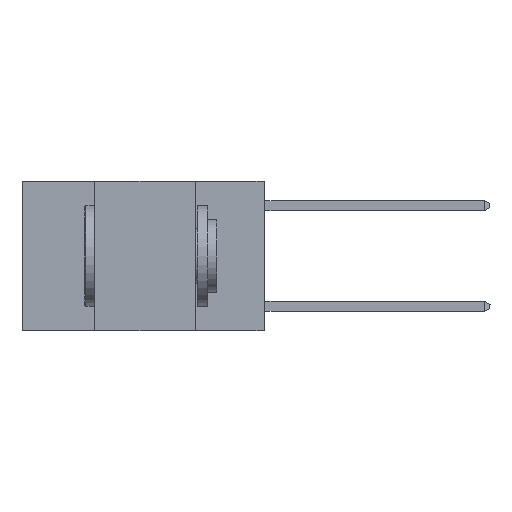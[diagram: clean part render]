
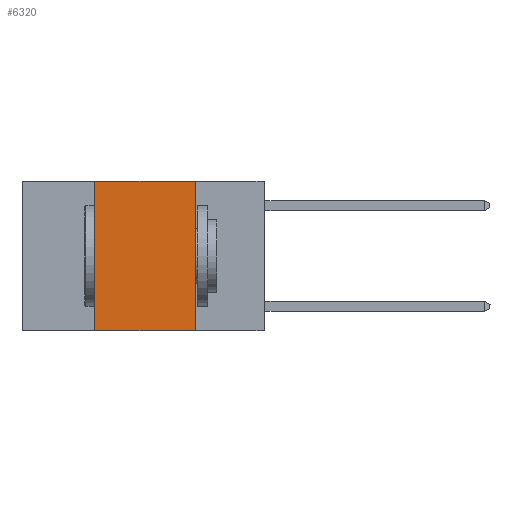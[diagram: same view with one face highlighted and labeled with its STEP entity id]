
A CAD part, left-side view. The second image highlights one B-rep face of the part: STEP entity #6320.
In plain terms, the highlighted planar face has unit normal (-1, 0, 0).
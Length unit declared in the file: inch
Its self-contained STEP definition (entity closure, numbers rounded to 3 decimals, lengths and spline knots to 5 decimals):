
#85 = VERTEX_POINT ( 'NONE', #10490 ) ;
#444 = DIRECTION ( 'NONE',  ( 0., 0., 1. ) ) ;
#3487 = EDGE_CURVE ( 'NONE', #22617, #15120, #13695, .T. ) ;
#5264 = CARTESIAN_POINT ( 'NONE',  ( 0., 0.42, 0. ) ) ;
#6052 = DIRECTION ( 'NONE',  ( 0., 0., -1. ) ) ;
#6320 = ADVANCED_FACE ( 'NONE', ( #25575 ), #9406, .F. ) ;
#7021 = CARTESIAN_POINT ( 'NONE',  ( 0., 0.6, 0. ) ) ;
#7198 = VECTOR ( 'NONE', #7482, 39.37008 ) ;
#7482 = DIRECTION ( 'NONE',  ( 0., -1., 0. ) ) ;
#8416 = CARTESIAN_POINT ( 'NONE',  ( 0., 0.6, 0. ) ) ;
#8564 = VECTOR ( 'NONE', #22892, 39.37008 ) ;
#9406 = PLANE ( 'NONE',  #19676 ) ;
#9510 = DIRECTION ( 'NONE',  ( 0., 0., -1. ) ) ;
#9922 = VECTOR ( 'NONE', #6052, 39.37008 ) ;
#10490 = CARTESIAN_POINT ( 'NONE',  ( 0., 0.17, 0. ) ) ;
#12734 = LINE ( 'NONE', #8416, #8564 ) ;
#13312 = CARTESIAN_POINT ( 'NONE',  ( 0., 0.17, 0. ) ) ;
#13695 = LINE ( 'NONE', #24418, #7198 ) ;
#15120 = VERTEX_POINT ( 'NONE', #24151 ) ;
#16175 = EDGE_CURVE ( 'NONE', #22973, #85, #12734, .T. ) ;
#16579 = EDGE_CURVE ( 'NONE', #22617, #22973, #19876, .T. ) ;
#17135 = ORIENTED_EDGE ( 'NONE', *, *, #16175, .F. ) ;
#17879 = ORIENTED_EDGE ( 'NONE', *, *, #16579, .F. ) ;
#19676 = AXIS2_PLACEMENT_3D ( 'NONE', #7021, #23963, #9510 ) ;
#19876 = LINE ( 'NONE', #5264, #25532 ) ;
#22008 = LINE ( 'NONE', #13312, #9922 ) ;
#22018 = ORIENTED_EDGE ( 'NONE', *, *, #29453, .F. ) ;
#22617 = VERTEX_POINT ( 'NONE', #30393 ) ;
#22892 = DIRECTION ( 'NONE',  ( 0., -1., 0. ) ) ;
#22973 = VERTEX_POINT ( 'NONE', #26907 ) ;
#23963 = DIRECTION ( 'NONE',  ( 1., 0., 0. ) ) ;
#24151 = CARTESIAN_POINT ( 'NONE',  ( 0., 0.17, -0.37 ) ) ;
#24350 = EDGE_LOOP ( 'NONE', ( #22018, #17135, #17879, #25033 ) ) ;
#24418 = CARTESIAN_POINT ( 'NONE',  ( 0., 0.6, -0.37 ) ) ;
#25033 = ORIENTED_EDGE ( 'NONE', *, *, #3487, .T. ) ;
#25532 = VECTOR ( 'NONE', #444, 39.37008 ) ;
#25575 = FACE_OUTER_BOUND ( 'NONE', #24350, .T. ) ;
#26907 = CARTESIAN_POINT ( 'NONE',  ( 0., 0.42, 0. ) ) ;
#29453 = EDGE_CURVE ( 'NONE', #85, #15120, #22008, .T. ) ;
#30393 = CARTESIAN_POINT ( 'NONE',  ( 0., 0.42, -0.37 ) ) ;
